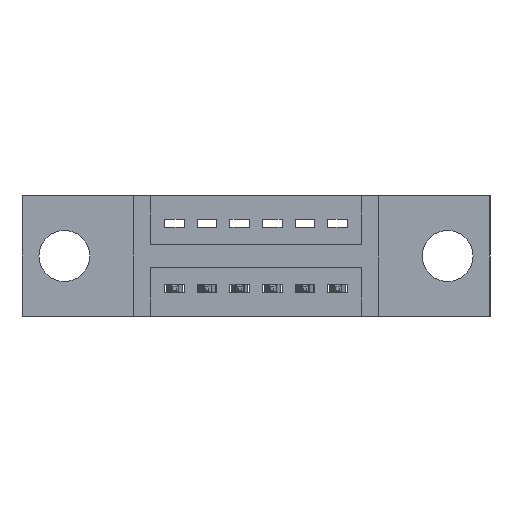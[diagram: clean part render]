
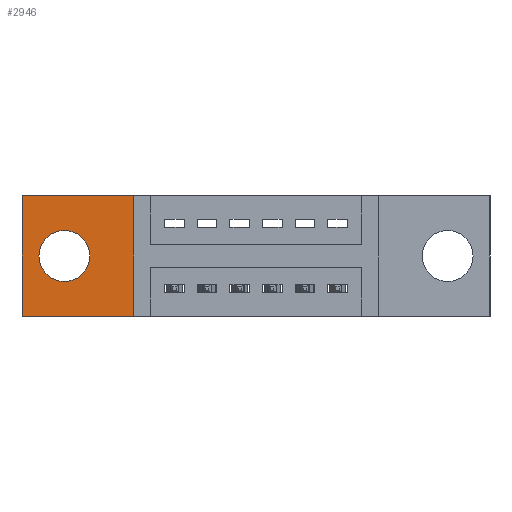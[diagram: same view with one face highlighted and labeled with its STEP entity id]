
A CAD part, front view. The second image highlights one B-rep face of the part: STEP entity #2946.
In plain terms, the highlighted planar face has unit normal (0, -1, 0).
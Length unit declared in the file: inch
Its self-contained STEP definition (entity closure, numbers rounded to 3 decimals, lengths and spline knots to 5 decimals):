
#45 = DIRECTION ( 'NONE',  ( 0., 0., 1. ) ) ;
#59 = DIRECTION ( 'NONE',  ( 0., -1., 0. ) ) ;
#454 = LINE ( 'NONE', #3610, #2713 ) ;
#654 = EDGE_CURVE ( 'NONE', #854, #4205, #9768, .T. ) ;
#854 = VERTEX_POINT ( 'NONE', #5486 ) ;
#1108 = EDGE_LOOP ( 'NONE', ( #2044, #5049, #6774, #3605 ) ) ;
#1129 = ORIENTED_EDGE ( 'NONE', *, *, #8067, .F. ) ;
#1210 = EDGE_CURVE ( 'NONE', #4205, #5459, #454, .T. ) ;
#1286 = CARTESIAN_POINT ( 'NONE',  ( 0.13, 0.17, -0.185 ) ) ;
#1742 = VERTEX_POINT ( 'NONE', #4686 ) ;
#2044 = ORIENTED_EDGE ( 'NONE', *, *, #654, .T. ) ;
#2175 = DIRECTION ( 'NONE',  ( 0., -1., 0. ) ) ;
#2713 = VECTOR ( 'NONE', #7486, 39.37008 ) ;
#2819 = VERTEX_POINT ( 'NONE', #6790 ) ;
#2946 = ADVANCED_FACE ( 'NONE', ( #3156, #3106 ), #7905, .T. ) ;
#3106 = FACE_OUTER_BOUND ( 'NONE', #1108, .T. ) ;
#3156 = FACE_BOUND ( 'NONE', #3566, .T. ) ;
#3282 = VERTEX_POINT ( 'NONE', #9089 ) ;
#3295 = AXIS2_PLACEMENT_3D ( 'NONE', #1286, #2175, #9785 ) ;
#3413 = LINE ( 'NONE', #7438, #5734 ) ;
#3433 = VECTOR ( 'NONE', #45, 39.37008 ) ;
#3566 = EDGE_LOOP ( 'NONE', ( #5203, #1129 ) ) ;
#3605 = ORIENTED_EDGE ( 'NONE', *, *, #8828, .T. ) ;
#3610 = CARTESIAN_POINT ( 'NONE',  ( 0., 0.17, -0.37 ) ) ;
#3637 = DIRECTION ( 'NONE',  ( 0., -1., 0. ) ) ;
#4205 = VERTEX_POINT ( 'NONE', #7954 ) ;
#4244 = CARTESIAN_POINT ( 'NONE',  ( 0.13, 0.17, -0.185 ) ) ;
#4686 = CARTESIAN_POINT ( 'NONE',  ( 0.3425, 0.17, 0. ) ) ;
#5049 = ORIENTED_EDGE ( 'NONE', *, *, #1210, .T. ) ;
#5203 = ORIENTED_EDGE ( 'NONE', *, *, #9305, .F. ) ;
#5350 = CARTESIAN_POINT ( 'NONE',  ( 0.3425, 0.17, -0.37 ) ) ;
#5366 = CARTESIAN_POINT ( 'NONE',  ( 0.3425, 0.17, 0. ) ) ;
#5459 = VERTEX_POINT ( 'NONE', #5350 ) ;
#5486 = CARTESIAN_POINT ( 'NONE',  ( 0., 0.17, 0. ) ) ;
#5639 = VECTOR ( 'NONE', #8864, 39.37008 ) ;
#5719 = CIRCLE ( 'NONE', #6825, 0.078 ) ;
#5734 = VECTOR ( 'NONE', #9610, 39.37008 ) ;
#6011 = DIRECTION ( 'NONE',  ( 0., 0., -1. ) ) ;
#6515 = CIRCLE ( 'NONE', #3295, 0.078 ) ;
#6596 = CARTESIAN_POINT ( 'NONE',  ( 0., 0.17, 0. ) ) ;
#6774 = ORIENTED_EDGE ( 'NONE', *, *, #7284, .T. ) ;
#6790 = CARTESIAN_POINT ( 'NONE',  ( 0.13, 0.17, -0.107 ) ) ;
#6825 = AXIS2_PLACEMENT_3D ( 'NONE', #4244, #3637, #6011 ) ;
#7284 = EDGE_CURVE ( 'NONE', #5459, #1742, #9289, .T. ) ;
#7438 = CARTESIAN_POINT ( 'NONE',  ( 0., 0.17, 0. ) ) ;
#7486 = DIRECTION ( 'NONE',  ( 1., 0., 0. ) ) ;
#7544 = AXIS2_PLACEMENT_3D ( 'NONE', #7747, #59, #8602 ) ;
#7747 = CARTESIAN_POINT ( 'NONE',  ( 0., 0.17, -0.37 ) ) ;
#7905 = PLANE ( 'NONE',  #7544 ) ;
#7954 = CARTESIAN_POINT ( 'NONE',  ( 0., 0.17, -0.37 ) ) ;
#8067 = EDGE_CURVE ( 'NONE', #3282, #2819, #5719, .T. ) ;
#8602 = DIRECTION ( 'NONE',  ( 0., 0., -1. ) ) ;
#8828 = EDGE_CURVE ( 'NONE', #1742, #854, #3413, .T. ) ;
#8864 = DIRECTION ( 'NONE',  ( 0., 0., -1. ) ) ;
#9089 = CARTESIAN_POINT ( 'NONE',  ( 0.13, 0.17, -0.263 ) ) ;
#9289 = LINE ( 'NONE', #5366, #3433 ) ;
#9305 = EDGE_CURVE ( 'NONE', #2819, #3282, #6515, .T. ) ;
#9610 = DIRECTION ( 'NONE',  ( -1., 0., 0. ) ) ;
#9768 = LINE ( 'NONE', #6596, #5639 ) ;
#9785 = DIRECTION ( 'NONE',  ( 0., 0., -1. ) ) ;
